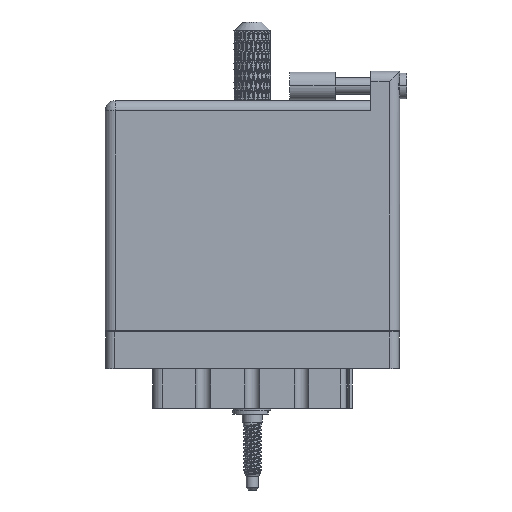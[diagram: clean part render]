
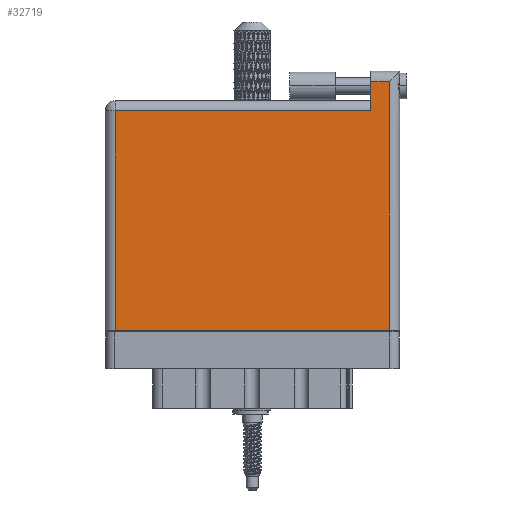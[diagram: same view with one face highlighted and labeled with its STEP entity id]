
A CAD part, front view. The second image highlights one B-rep face of the part: STEP entity #32719.
In plain terms, the highlighted face is planar.
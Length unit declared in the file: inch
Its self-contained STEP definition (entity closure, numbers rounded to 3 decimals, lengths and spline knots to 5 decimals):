
#1109 = CARTESIAN_POINT ( 'NONE',  ( 1.811, 1.696, 0. ) ) ;
#1942 = LINE ( 'NONE', #35624, #102435 ) ;
#2515 = CARTESIAN_POINT ( 'NONE',  ( 1.938, 1.696, 0. ) ) ;
#3030 = DIRECTION ( 'NONE',  ( 0., 1., 0. ) ) ;
#5431 = CARTESIAN_POINT ( 'NONE',  ( 0., 1.496, 0. ) ) ;
#6279 = PLANE ( 'NONE',  #74281 ) ;
#11202 = LINE ( 'NONE', #5431, #75645 ) ;
#11963 = LINE ( 'NONE', #70585, #80240 ) ;
#12685 = ORIENTED_EDGE ( 'NONE', *, *, #73353, .T. ) ;
#12869 = DIRECTION ( 'NONE',  ( 0., -1., 0. ) ) ;
#16224 = LINE ( 'NONE', #93402, #18846 ) ;
#18846 = VECTOR ( 'NONE', #3030, 39.37008 ) ;
#20095 = VECTOR ( 'NONE', #55285, 39.37008 ) ;
#21317 = DIRECTION ( 'NONE',  ( 0., -1., 0. ) ) ;
#24004 = EDGE_CURVE ( 'NONE', #74297, #44703, #16224, .T. ) ;
#25847 = LINE ( 'NONE', #102906, #43936 ) ;
#26232 = EDGE_CURVE ( 'NONE', #44703, #47359, #1942, .T. ) ;
#27235 = EDGE_CURVE ( 'NONE', #93000, #91779, #11963, .T. ) ;
#30076 = ORIENTED_EDGE ( 'NONE', *, *, #26232, .T. ) ;
#30468 = CARTESIAN_POINT ( 'NONE',  ( 1.811, 1.496, 0. ) ) ;
#31019 = CARTESIAN_POINT ( 'NONE',  ( 0.07, 1.496, 0. ) ) ;
#32211 = CARTESIAN_POINT ( 'NONE',  ( 0., 1.566, 0. ) ) ;
#32719 = ADVANCED_FACE ( 'NONE', ( #69405 ), #6279, .F. ) ;
#34243 = EDGE_CURVE ( 'NONE', #45290, #93000, #11202, .T. ) ;
#35624 = CARTESIAN_POINT ( 'NONE',  ( 0., 1.696, 0. ) ) ;
#38073 = LINE ( 'NONE', #47065, #20095 ) ;
#40822 = DIRECTION ( 'NONE',  ( -1., 0., 0. ) ) ;
#42447 = EDGE_LOOP ( 'NONE', ( #12685, #67039, #30076, #106568, #102629, #95606 ) ) ;
#43200 = DIRECTION ( 'NONE',  ( -1., 0., 0. ) ) ;
#43936 = VECTOR ( 'NONE', #12869, 39.37008 ) ;
#44703 = VERTEX_POINT ( 'NONE', #2515 ) ;
#45290 = VERTEX_POINT ( 'NONE', #30468 ) ;
#47065 = CARTESIAN_POINT ( 'NONE',  ( 0., 0., 0. ) ) ;
#47359 = VERTEX_POINT ( 'NONE', #1109 ) ;
#52650 = CARTESIAN_POINT ( 'NONE',  ( 1.938, 0., 0. ) ) ;
#54123 = CARTESIAN_POINT ( 'NONE',  ( 0.07, 0., 0. ) ) ;
#55285 = DIRECTION ( 'NONE',  ( 1., 0., 0. ) ) ;
#55799 = DIRECTION ( 'NONE',  ( -1., 0., 0. ) ) ;
#56990 = DIRECTION ( 'NONE',  ( 0., 0., -1. ) ) ;
#67039 = ORIENTED_EDGE ( 'NONE', *, *, #24004, .T. ) ;
#69405 = FACE_OUTER_BOUND ( 'NONE', #42447, .T. ) ;
#70585 = CARTESIAN_POINT ( 'NONE',  ( 0.07, 0., 0. ) ) ;
#73353 = EDGE_CURVE ( 'NONE', #91779, #74297, #38073, .T. ) ;
#74281 = AXIS2_PLACEMENT_3D ( 'NONE', #32211, #56990, #40822 ) ;
#74297 = VERTEX_POINT ( 'NONE', #52650 ) ;
#75645 = VECTOR ( 'NONE', #55799, 39.37008 ) ;
#80240 = VECTOR ( 'NONE', #21317, 39.37008 ) ;
#91324 = EDGE_CURVE ( 'NONE', #47359, #45290, #25847, .T. ) ;
#91779 = VERTEX_POINT ( 'NONE', #54123 ) ;
#93000 = VERTEX_POINT ( 'NONE', #31019 ) ;
#93402 = CARTESIAN_POINT ( 'NONE',  ( 1.938, 1.766, 0. ) ) ;
#95606 = ORIENTED_EDGE ( 'NONE', *, *, #27235, .T. ) ;
#102435 = VECTOR ( 'NONE', #43200, 39.37008 ) ;
#102629 = ORIENTED_EDGE ( 'NONE', *, *, #34243, .T. ) ;
#102906 = CARTESIAN_POINT ( 'NONE',  ( 1.811, 1.766, 0. ) ) ;
#106568 = ORIENTED_EDGE ( 'NONE', *, *, #91324, .T. ) ;
